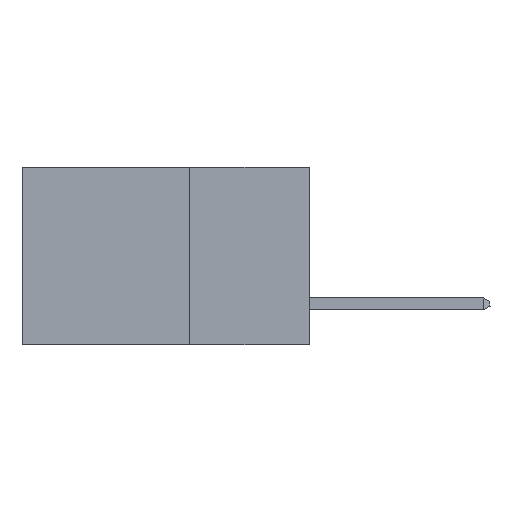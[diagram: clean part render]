
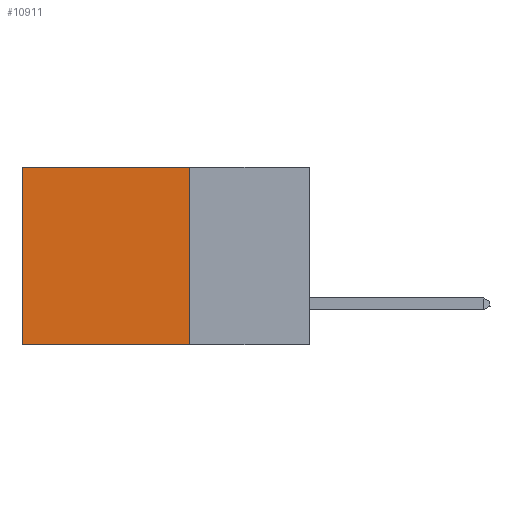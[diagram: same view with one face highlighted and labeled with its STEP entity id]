
A CAD part, left-side view. The second image highlights one B-rep face of the part: STEP entity #10911.
In plain terms, the highlighted planar face has unit normal (-1, 0, 0).
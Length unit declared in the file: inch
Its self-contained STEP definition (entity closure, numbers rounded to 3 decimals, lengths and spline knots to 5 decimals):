
#1293 = VECTOR ( 'NONE', #42344, 39.37008 ) ;
#1664 = DIRECTION ( 'NONE',  ( 1., 0., 0. ) ) ;
#1759 = LINE ( 'NONE', #21956, #4526 ) ;
#2060 = FACE_OUTER_BOUND ( 'NONE', #20688, .T. ) ;
#2401 = VERTEX_POINT ( 'NONE', #20428 ) ;
#4526 = VECTOR ( 'NONE', #25801, 39.37008 ) ;
#5172 = EDGE_CURVE ( 'NONE', #29849, #33505, #25153, .T. ) ;
#5422 = ORIENTED_EDGE ( 'NONE', *, *, #7613, .F. ) ;
#6674 = DIRECTION ( 'NONE',  ( 0., 1., 0. ) ) ;
#7613 = EDGE_CURVE ( 'NONE', #33505, #22703, #1759, .T. ) ;
#9146 = CARTESIAN_POINT ( 'NONE',  ( 0.2875, 0.6, -0.37 ) ) ;
#10911 = ADVANCED_FACE ( 'NONE', ( #2060 ), #22941, .F. ) ;
#11024 = AXIS2_PLACEMENT_3D ( 'NONE', #33126, #1664, #22286 ) ;
#12351 = LINE ( 'NONE', #31308, #32292 ) ;
#12394 = ORIENTED_EDGE ( 'NONE', *, *, #14292, .T. ) ;
#12701 = CARTESIAN_POINT ( 'NONE',  ( 0.2875, 0.25, 0. ) ) ;
#14094 = ORIENTED_EDGE ( 'NONE', *, *, #42352, .T. ) ;
#14292 = EDGE_CURVE ( 'NONE', #2401, #22703, #28501, .T. ) ;
#20428 = CARTESIAN_POINT ( 'NONE',  ( 0.2875, 0.6, 0. ) ) ;
#20688 = EDGE_LOOP ( 'NONE', ( #12394, #5422, #41747, #14094 ) ) ;
#21956 = CARTESIAN_POINT ( 'NONE',  ( 0.2875, 0.25, -0.37 ) ) ;
#22286 = DIRECTION ( 'NONE',  ( 0., 0., -1. ) ) ;
#22703 = VERTEX_POINT ( 'NONE', #9146 ) ;
#22941 = PLANE ( 'NONE',  #11024 ) ;
#25153 = LINE ( 'NONE', #12701, #42837 ) ;
#25801 = DIRECTION ( 'NONE',  ( 0., 1., 0. ) ) ;
#28344 = CARTESIAN_POINT ( 'NONE',  ( 0.2875, 0.6, 0. ) ) ;
#28501 = LINE ( 'NONE', #28344, #1293 ) ;
#29684 = DIRECTION ( 'NONE',  ( 0., 0., -1. ) ) ;
#29849 = VERTEX_POINT ( 'NONE', #43985 ) ;
#31308 = CARTESIAN_POINT ( 'NONE',  ( 0.2875, 0.25, 0. ) ) ;
#32292 = VECTOR ( 'NONE', #6674, 39.37008 ) ;
#33126 = CARTESIAN_POINT ( 'NONE',  ( 0.2875, 0.25, 0. ) ) ;
#33505 = VERTEX_POINT ( 'NONE', #35960 ) ;
#35960 = CARTESIAN_POINT ( 'NONE',  ( 0.2875, 0.25, -0.37 ) ) ;
#41747 = ORIENTED_EDGE ( 'NONE', *, *, #5172, .F. ) ;
#42344 = DIRECTION ( 'NONE',  ( 0., 0., -1. ) ) ;
#42352 = EDGE_CURVE ( 'NONE', #29849, #2401, #12351, .T. ) ;
#42837 = VECTOR ( 'NONE', #29684, 39.37008 ) ;
#43985 = CARTESIAN_POINT ( 'NONE',  ( 0.2875, 0.25, 0. ) ) ;
